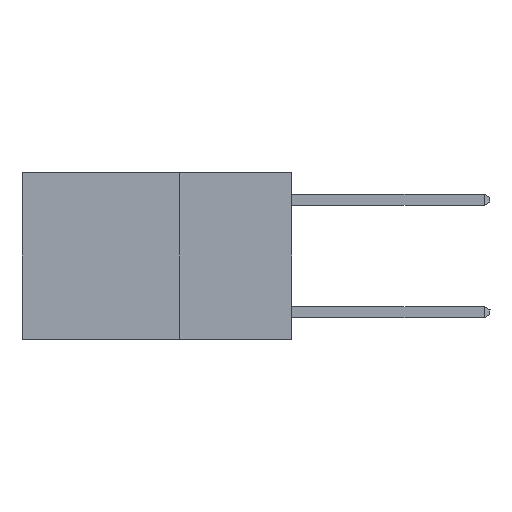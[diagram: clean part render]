
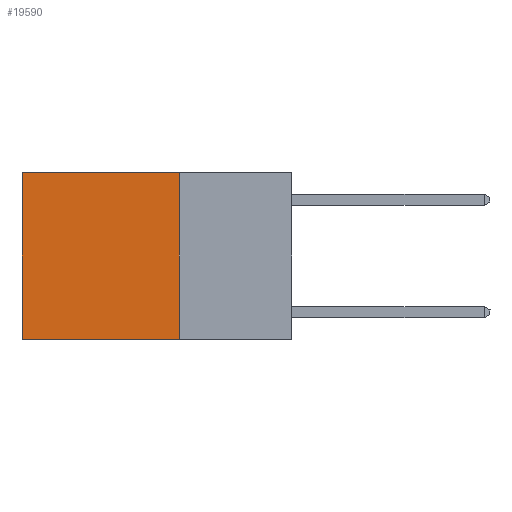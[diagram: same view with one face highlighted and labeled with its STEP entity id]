
A CAD part, left-side view. The second image highlights one B-rep face of the part: STEP entity #19590.
In plain terms, the highlighted planar face has unit normal (-1, 0, 0).
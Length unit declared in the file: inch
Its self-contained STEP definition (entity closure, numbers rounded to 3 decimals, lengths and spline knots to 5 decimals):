
#599 = CARTESIAN_POINT ( 'NONE',  ( 0.2625, 0.6, 0. ) ) ;
#861 = VERTEX_POINT ( 'NONE', #12810 ) ;
#1005 = VECTOR ( 'NONE', #12706, 39.37008 ) ;
#2199 = DIRECTION ( 'NONE',  ( 0., 0., -1. ) ) ;
#3236 = ORIENTED_EDGE ( 'NONE', *, *, #19068, .T. ) ;
#3330 = CARTESIAN_POINT ( 'NONE',  ( 0.2625, 0.25, -0.37 ) ) ;
#3546 = EDGE_LOOP ( 'NONE', ( #3919, #7282, #4258, #3236 ) ) ;
#3919 = ORIENTED_EDGE ( 'NONE', *, *, #4256, .T. ) ;
#4005 = EDGE_CURVE ( 'NONE', #10414, #861, #15457, .T. ) ;
#4256 = EDGE_CURVE ( 'NONE', #9874, #861, #16370, .T. ) ;
#4258 = ORIENTED_EDGE ( 'NONE', *, *, #14411, .F. ) ;
#4414 = PLANE ( 'NONE',  #15018 ) ;
#5416 = LINE ( 'NONE', #14203, #1005 ) ;
#5994 = CARTESIAN_POINT ( 'NONE',  ( 0.2625, 0.25, 0. ) ) ;
#6981 = CARTESIAN_POINT ( 'NONE',  ( 0.2625, 0.25, -0.37 ) ) ;
#7119 = VECTOR ( 'NONE', #14515, 39.37008 ) ;
#7282 = ORIENTED_EDGE ( 'NONE', *, *, #4005, .F. ) ;
#7692 = DIRECTION ( 'NONE',  ( 1., 0., 0. ) ) ;
#9874 = VERTEX_POINT ( 'NONE', #599 ) ;
#10100 = DIRECTION ( 'NONE',  ( 0., 0., -1. ) ) ;
#10414 = VERTEX_POINT ( 'NONE', #6981 ) ;
#12037 = LINE ( 'NONE', #13167, #16932 ) ;
#12372 = VERTEX_POINT ( 'NONE', #5994 ) ;
#12382 = VECTOR ( 'NONE', #2199, 39.37008 ) ;
#12706 = DIRECTION ( 'NONE',  ( 0., 1., 0. ) ) ;
#12810 = CARTESIAN_POINT ( 'NONE',  ( 0.2625, 0.6, -0.37 ) ) ;
#13167 = CARTESIAN_POINT ( 'NONE',  ( 0.2625, 0.25, 0. ) ) ;
#14203 = CARTESIAN_POINT ( 'NONE',  ( 0.2625, 0.25, 0. ) ) ;
#14411 = EDGE_CURVE ( 'NONE', #12372, #10414, #12037, .T. ) ;
#14515 = DIRECTION ( 'NONE',  ( 0., 1., 0. ) ) ;
#14607 = FACE_OUTER_BOUND ( 'NONE', #3546, .T. ) ;
#15018 = AXIS2_PLACEMENT_3D ( 'NONE', #16951, #7692, #18339 ) ;
#15457 = LINE ( 'NONE', #3330, #7119 ) ;
#16370 = LINE ( 'NONE', #19264, #12382 ) ;
#16932 = VECTOR ( 'NONE', #10100, 39.37008 ) ;
#16951 = CARTESIAN_POINT ( 'NONE',  ( 0.2625, 0.25, 0. ) ) ;
#18339 = DIRECTION ( 'NONE',  ( 0., 0., -1. ) ) ;
#19068 = EDGE_CURVE ( 'NONE', #12372, #9874, #5416, .T. ) ;
#19264 = CARTESIAN_POINT ( 'NONE',  ( 0.2625, 0.6, 0. ) ) ;
#19590 = ADVANCED_FACE ( 'NONE', ( #14607 ), #4414, .F. ) ;
